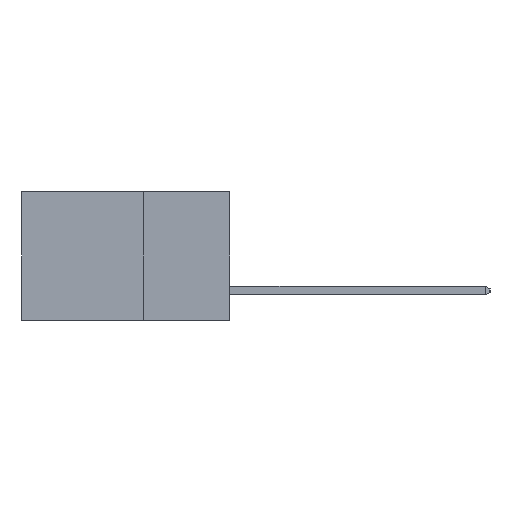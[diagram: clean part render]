
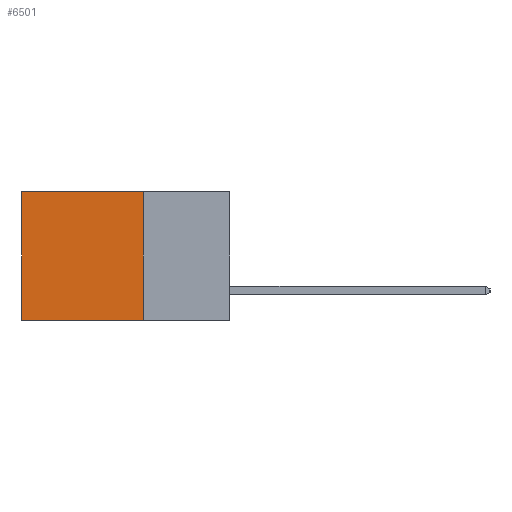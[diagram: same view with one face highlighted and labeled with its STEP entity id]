
A CAD part, left-side view. The second image highlights one B-rep face of the part: STEP entity #6501.
In plain terms, the highlighted planar face has unit normal (-1, 0, 0).
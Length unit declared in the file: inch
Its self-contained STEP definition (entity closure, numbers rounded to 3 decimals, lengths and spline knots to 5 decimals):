
#762 = ORIENTED_EDGE ( 'NONE', *, *, #25277, .T. ) ;
#992 = DIRECTION ( 'NONE',  ( 0., 0., -1. ) ) ;
#1065 = VERTEX_POINT ( 'NONE', #19053 ) ;
#2371 = VERTEX_POINT ( 'NONE', #14459 ) ;
#3974 = LINE ( 'NONE', #15282, #24741 ) ;
#5072 = FACE_OUTER_BOUND ( 'NONE', #9786, .T. ) ;
#5996 = VERTEX_POINT ( 'NONE', #10705 ) ;
#6163 = EDGE_CURVE ( 'NONE', #2371, #14622, #14625, .T. ) ;
#6335 = DIRECTION ( 'NONE',  ( 0., 0., -1. ) ) ;
#6501 = ADVANCED_FACE ( 'NONE', ( #5072 ), #7097, .F. ) ;
#6534 = VECTOR ( 'NONE', #9288, 39.37008 ) ;
#6610 = DIRECTION ( 'NONE',  ( 1., 0., 0. ) ) ;
#6924 = ORIENTED_EDGE ( 'NONE', *, *, #11684, .F. ) ;
#7097 = PLANE ( 'NONE',  #15057 ) ;
#7252 = CARTESIAN_POINT ( 'NONE',  ( 0.298, 0.6, 0. ) ) ;
#7289 = DIRECTION ( 'NONE',  ( 0., 1., 0. ) ) ;
#7779 = CARTESIAN_POINT ( 'NONE',  ( 0.298, 0.25, 0. ) ) ;
#9188 = CARTESIAN_POINT ( 'NONE',  ( 0.298, 0.25, 0. ) ) ;
#9288 = DIRECTION ( 'NONE',  ( 0., 0., -1. ) ) ;
#9786 = EDGE_LOOP ( 'NONE', ( #15683, #15197, #6924, #762 ) ) ;
#10690 = VECTOR ( 'NONE', #992, 39.37008 ) ;
#10705 = CARTESIAN_POINT ( 'NONE',  ( 0.298, 0.6, 0. ) ) ;
#11684 = EDGE_CURVE ( 'NONE', #1065, #2371, #15476, .T. ) ;
#11996 = CARTESIAN_POINT ( 'NONE',  ( 0.298, 0.6, -0.37 ) ) ;
#13479 = CARTESIAN_POINT ( 'NONE',  ( 0.298, 0.25, -0.37 ) ) ;
#14459 = CARTESIAN_POINT ( 'NONE',  ( 0.298, 0.25, -0.37 ) ) ;
#14622 = VERTEX_POINT ( 'NONE', #11996 ) ;
#14625 = LINE ( 'NONE', #13479, #18750 ) ;
#15057 = AXIS2_PLACEMENT_3D ( 'NONE', #7779, #6610, #6335 ) ;
#15197 = ORIENTED_EDGE ( 'NONE', *, *, #6163, .F. ) ;
#15282 = CARTESIAN_POINT ( 'NONE',  ( 0.298, 0.25, 0. ) ) ;
#15476 = LINE ( 'NONE', #9188, #10690 ) ;
#15683 = ORIENTED_EDGE ( 'NONE', *, *, #21073, .T. ) ;
#16377 = DIRECTION ( 'NONE',  ( 0., 1., 0. ) ) ;
#18750 = VECTOR ( 'NONE', #16377, 39.37008 ) ;
#19053 = CARTESIAN_POINT ( 'NONE',  ( 0.298, 0.25, 0. ) ) ;
#21073 = EDGE_CURVE ( 'NONE', #5996, #14622, #22583, .T. ) ;
#22583 = LINE ( 'NONE', #7252, #6534 ) ;
#24741 = VECTOR ( 'NONE', #7289, 39.37008 ) ;
#25277 = EDGE_CURVE ( 'NONE', #1065, #5996, #3974, .T. ) ;
